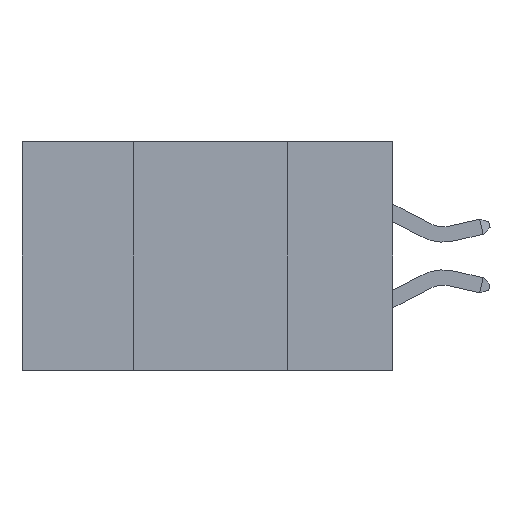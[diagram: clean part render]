
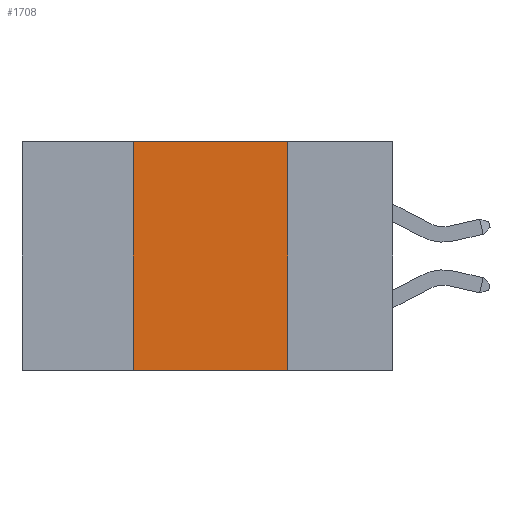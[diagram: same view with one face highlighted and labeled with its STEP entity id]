
A CAD part, left-side view. The second image highlights one B-rep face of the part: STEP entity #1708.
In plain terms, the highlighted planar face has unit normal (-1, 0, 0).
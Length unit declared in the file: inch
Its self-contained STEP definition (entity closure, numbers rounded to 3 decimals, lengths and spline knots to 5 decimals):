
#90 = CARTESIAN_POINT ( 'NONE',  ( 0., 0.6, 0. ) ) ;
#464 = VECTOR ( 'NONE', #18941, 39.37008 ) ;
#1708 = ADVANCED_FACE ( 'NONE', ( #13083 ), #18629, .F. ) ;
#1859 = CARTESIAN_POINT ( 'NONE',  ( 0., 0.6, 0. ) ) ;
#2420 = EDGE_CURVE ( 'NONE', #3224, #17775, #6105, .T. ) ;
#2541 = CARTESIAN_POINT ( 'NONE',  ( 0., 0.6, -0.37 ) ) ;
#2792 = VECTOR ( 'NONE', #17598, 39.37008 ) ;
#3224 = VERTEX_POINT ( 'NONE', #22533 ) ;
#3693 = DIRECTION ( 'NONE',  ( 1., 0., 0. ) ) ;
#3721 = CARTESIAN_POINT ( 'NONE',  ( 0., 0.17, 0. ) ) ;
#3854 = LINE ( 'NONE', #90, #5032 ) ;
#5032 = VECTOR ( 'NONE', #9136, 39.37008 ) ;
#5328 = DIRECTION ( 'NONE',  ( 0., 0., -1. ) ) ;
#5422 = DIRECTION ( 'NONE',  ( 0., 0., -1. ) ) ;
#5687 = ORIENTED_EDGE ( 'NONE', *, *, #2420, .F. ) ;
#6105 = LINE ( 'NONE', #13874, #464 ) ;
#6440 = EDGE_CURVE ( 'NONE', #17775, #18861, #3854, .T. ) ;
#6882 = ORIENTED_EDGE ( 'NONE', *, *, #7492, .T. ) ;
#7492 = EDGE_CURVE ( 'NONE', #3224, #11674, #19184, .T. ) ;
#9136 = DIRECTION ( 'NONE',  ( 0., -1., 0. ) ) ;
#9689 = VECTOR ( 'NONE', #5328, 39.37008 ) ;
#10182 = ORIENTED_EDGE ( 'NONE', *, *, #6440, .F. ) ;
#11013 = EDGE_LOOP ( 'NONE', ( #21399, #10182, #5687, #6882 ) ) ;
#11241 = CARTESIAN_POINT ( 'NONE',  ( 0., 0.42, 0. ) ) ;
#11674 = VERTEX_POINT ( 'NONE', #12082 ) ;
#12082 = CARTESIAN_POINT ( 'NONE',  ( 0., 0.17, -0.37 ) ) ;
#13083 = FACE_OUTER_BOUND ( 'NONE', #11013, .T. ) ;
#13874 = CARTESIAN_POINT ( 'NONE',  ( 0., 0.42, 0. ) ) ;
#14767 = AXIS2_PLACEMENT_3D ( 'NONE', #1859, #3693, #5422 ) ;
#15130 = EDGE_CURVE ( 'NONE', #18861, #11674, #16613, .T. ) ;
#16613 = LINE ( 'NONE', #3721, #9689 ) ;
#17598 = DIRECTION ( 'NONE',  ( 0., -1., 0. ) ) ;
#17775 = VERTEX_POINT ( 'NONE', #11241 ) ;
#18629 = PLANE ( 'NONE',  #14767 ) ;
#18861 = VERTEX_POINT ( 'NONE', #21565 ) ;
#18941 = DIRECTION ( 'NONE',  ( 0., 0., 1. ) ) ;
#19184 = LINE ( 'NONE', #2541, #2792 ) ;
#21399 = ORIENTED_EDGE ( 'NONE', *, *, #15130, .F. ) ;
#21565 = CARTESIAN_POINT ( 'NONE',  ( 0., 0.17, 0. ) ) ;
#22533 = CARTESIAN_POINT ( 'NONE',  ( 0., 0.42, -0.37 ) ) ;
